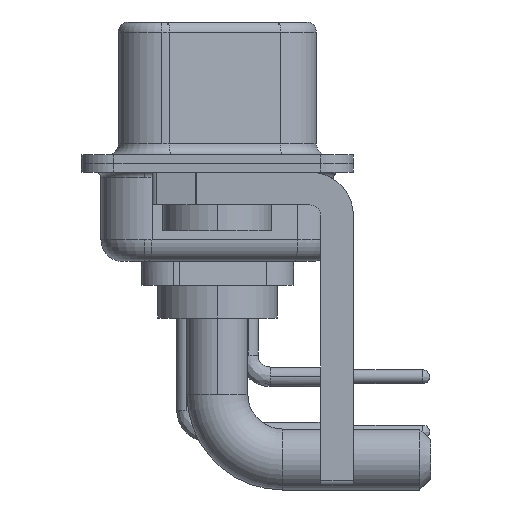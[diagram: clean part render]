
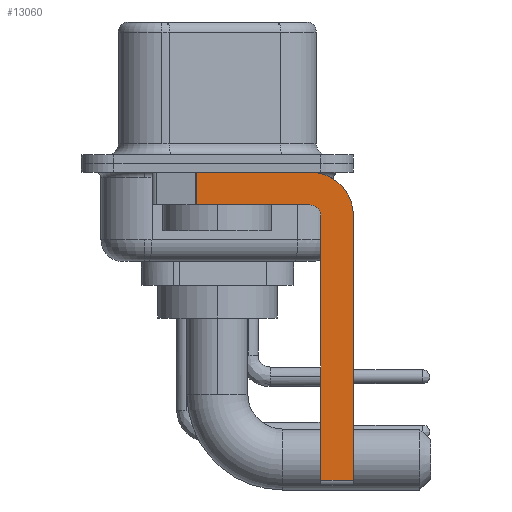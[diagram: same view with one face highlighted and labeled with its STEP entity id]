
A CAD part, left-side view. The second image highlights one B-rep face of the part: STEP entity #13060.
In plain terms, the highlighted planar face has unit normal (-1, 0, 0).
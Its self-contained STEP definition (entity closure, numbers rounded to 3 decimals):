
#196 = LINE ( 'NONE', #6481, #22517 ) ;
#373 = CARTESIAN_POINT ( 'NONE',  ( -2.9, -6.25, -14.55 ) ) ;
#435 = DIRECTION ( 'NONE',  ( 1., 0., 0. ) ) ;
#1340 = ORIENTED_EDGE ( 'NONE', *, *, #12212, .F. ) ;
#1704 = VECTOR ( 'NONE', #23721, 1000. ) ;
#1833 = LINE ( 'NONE', #10651, #8214 ) ;
#1897 = EDGE_CURVE ( 'NONE', #5061, #23573, #12772, .T. ) ;
#2861 = AXIS2_PLACEMENT_3D ( 'NONE', #25524, #4938, #22678 ) ;
#4046 = ORIENTED_EDGE ( 'NONE', *, *, #12094, .F. ) ;
#4938 = DIRECTION ( 'NONE',  ( 1., 0., 0. ) ) ;
#5061 = VERTEX_POINT ( 'NONE', #19162 ) ;
#5224 = AXIS2_PLACEMENT_3D ( 'NONE', #19054, #435, #9557 ) ;
#6481 = CARTESIAN_POINT ( 'NONE',  ( -2.9, 0.978, -1.9 ) ) ;
#7893 = DIRECTION ( 'NONE',  ( 0., 1., 0. ) ) ;
#8086 = CARTESIAN_POINT ( 'NONE',  ( -2.9, -6.25, -2.4 ) ) ;
#8214 = VECTOR ( 'NONE', #17482, 1000. ) ;
#8403 = ORIENTED_EDGE ( 'NONE', *, *, #25269, .T. ) ;
#8923 = DIRECTION ( 'NONE',  ( -1., 0., 0. ) ) ;
#9557 = DIRECTION ( 'NONE',  ( 0., 0., -1. ) ) ;
#9919 = DIRECTION ( 'NONE',  ( 0., -1., 0. ) ) ;
#10400 = ORIENTED_EDGE ( 'NONE', *, *, #19157, .T. ) ;
#10651 = CARTESIAN_POINT ( 'NONE',  ( -2.9, -4.75, -14.8 ) ) ;
#10881 = VECTOR ( 'NONE', #9919, 1000. ) ;
#12094 = EDGE_CURVE ( 'NONE', #20621, #17318, #1833, .T. ) ;
#12212 = EDGE_CURVE ( 'NONE', #23573, #15806, #22369, .T. ) ;
#12426 = EDGE_LOOP ( 'NONE', ( #25844, #8403, #22926, #28864, #4046, #10400, #15059, #1340 ) ) ;
#12607 = CARTESIAN_POINT ( 'NONE',  ( -2.9, -4.75, -14.55 ) ) ;
#12772 = LINE ( 'NONE', #21395, #20441 ) ;
#13060 = ADVANCED_FACE ( 'NONE', ( #23387 ), #27865, .F. ) ;
#14795 = LINE ( 'NONE', #8086, #1704 ) ;
#15059 = ORIENTED_EDGE ( 'NONE', *, *, #15966, .F. ) ;
#15806 = VERTEX_POINT ( 'NONE', #22984 ) ;
#15966 = EDGE_CURVE ( 'NONE', #15806, #19211, #14795, .T. ) ;
#16177 = CARTESIAN_POINT ( 'NONE',  ( -2.9, -4.25, -0.4 ) ) ;
#16580 = EDGE_CURVE ( 'NONE', #17318, #23008, #17437, .T. ) ;
#16746 = CARTESIAN_POINT ( 'NONE',  ( -2.9, -4.25, -14.55 ) ) ;
#17318 = VERTEX_POINT ( 'NONE', #18171 ) ;
#17437 = CIRCLE ( 'NONE', #27433, 0.5 ) ;
#17482 = DIRECTION ( 'NONE',  ( 0., 0., 1. ) ) ;
#18171 = CARTESIAN_POINT ( 'NONE',  ( -2.9, -4.75, -2.4 ) ) ;
#19054 = CARTESIAN_POINT ( 'NONE',  ( -2.9, -4.25, -2.4 ) ) ;
#19157 = EDGE_CURVE ( 'NONE', #20621, #19211, #21229, .T. ) ;
#19162 = CARTESIAN_POINT ( 'NONE',  ( -2.9, 0.978, -0.4 ) ) ;
#19211 = VERTEX_POINT ( 'NONE', #373 ) ;
#20441 = VECTOR ( 'NONE', #21684, 1000. ) ;
#20621 = VERTEX_POINT ( 'NONE', #12607 ) ;
#21229 = LINE ( 'NONE', #16746, #10881 ) ;
#21395 = CARTESIAN_POINT ( 'NONE',  ( -2.9, 3., -0.4 ) ) ;
#21684 = DIRECTION ( 'NONE',  ( 0., -1., 0. ) ) ;
#22323 = CARTESIAN_POINT ( 'NONE',  ( -2.9, -4.25, -1.9 ) ) ;
#22369 = CIRCLE ( 'NONE', #2861, 2. ) ;
#22517 = VECTOR ( 'NONE', #22859, 1000. ) ;
#22678 = DIRECTION ( 'NONE',  ( 0., 0., -1. ) ) ;
#22859 = DIRECTION ( 'NONE',  ( 0., 0., -1. ) ) ;
#22926 = ORIENTED_EDGE ( 'NONE', *, *, #25662, .F. ) ;
#22984 = CARTESIAN_POINT ( 'NONE',  ( -2.9, -6.25, -2.4 ) ) ;
#23008 = VERTEX_POINT ( 'NONE', #22323 ) ;
#23387 = FACE_OUTER_BOUND ( 'NONE', #12426, .T. ) ;
#23573 = VERTEX_POINT ( 'NONE', #16177 ) ;
#23721 = DIRECTION ( 'NONE',  ( 0., 0., -1. ) ) ;
#25269 = EDGE_CURVE ( 'NONE', #5061, #27758, #196, .T. ) ;
#25494 = CARTESIAN_POINT ( 'NONE',  ( -2.9, -4.25, -1.9 ) ) ;
#25524 = CARTESIAN_POINT ( 'NONE',  ( -2.9, -4.25, -2.4 ) ) ;
#25662 = EDGE_CURVE ( 'NONE', #23008, #27758, #28318, .T. ) ;
#25844 = ORIENTED_EDGE ( 'NONE', *, *, #1897, .F. ) ;
#27112 = DIRECTION ( 'NONE',  ( 0., 0., 1. ) ) ;
#27433 = AXIS2_PLACEMENT_3D ( 'NONE', #29341, #8923, #27112 ) ;
#27758 = VERTEX_POINT ( 'NONE', #28931 ) ;
#27865 = PLANE ( 'NONE',  #5224 ) ;
#28318 = LINE ( 'NONE', #25494, #29217 ) ;
#28864 = ORIENTED_EDGE ( 'NONE', *, *, #16580, .F. ) ;
#28931 = CARTESIAN_POINT ( 'NONE',  ( -2.9, 0.978, -1.9 ) ) ;
#29217 = VECTOR ( 'NONE', #7893, 1000. ) ;
#29341 = CARTESIAN_POINT ( 'NONE',  ( -2.9, -4.25, -2.4 ) ) ;
